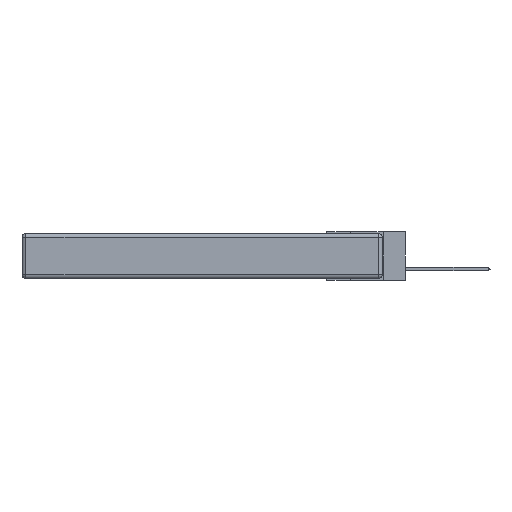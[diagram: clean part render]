
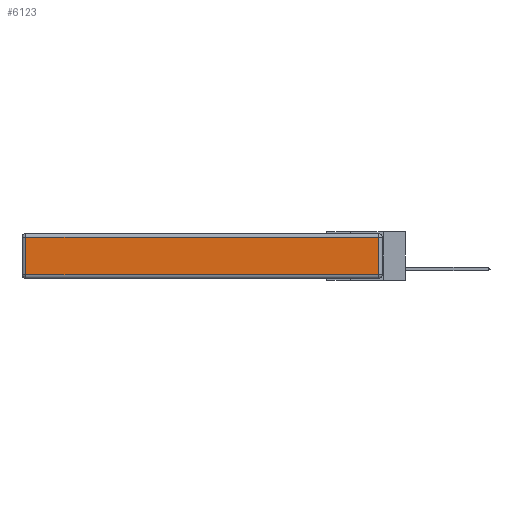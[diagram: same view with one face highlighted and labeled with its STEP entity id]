
A CAD part, left-side view. The second image highlights one B-rep face of the part: STEP entity #6123.
In plain terms, the highlighted planar face has unit normal (-1, 0, 0).
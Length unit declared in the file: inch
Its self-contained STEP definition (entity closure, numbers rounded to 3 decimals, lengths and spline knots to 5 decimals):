
#11 = AXIS2_PLACEMENT_3D ( 'NONE', #829, #14821, #4295 ) ;
#829 = CARTESIAN_POINT ( 'NONE',  ( 0., 0., -0.343 ) ) ;
#1125 = EDGE_LOOP ( 'NONE', ( #17814, #9909, #19989, #3002 ) ) ;
#2031 = VECTOR ( 'NONE', #16127, 39.37008 ) ;
#3002 = ORIENTED_EDGE ( 'NONE', *, *, #18448, .T. ) ;
#3499 = DIRECTION ( 'NONE',  ( 0., -1., 0. ) ) ;
#3679 = CARTESIAN_POINT ( 'NONE',  ( 0., 2.72, -0.313 ) ) ;
#4295 = DIRECTION ( 'NONE',  ( 0., 0., 1. ) ) ;
#5019 = EDGE_CURVE ( 'NONE', #17377, #13344, #14446, .T. ) ;
#5867 = PLANE ( 'NONE',  #11 ) ;
#6123 = ADVANCED_FACE ( 'NONE', ( #9942 ), #5867, .T. ) ;
#6393 = CARTESIAN_POINT ( 'NONE',  ( 0., 2.72, -0.03 ) ) ;
#8538 = VERTEX_POINT ( 'NONE', #3679 ) ;
#9721 = VECTOR ( 'NONE', #21737, 39.37008 ) ;
#9909 = ORIENTED_EDGE ( 'NONE', *, *, #11737, .T. ) ;
#9942 = FACE_OUTER_BOUND ( 'NONE', #1125, .T. ) ;
#10333 = CARTESIAN_POINT ( 'NONE',  ( 0., 2.72, -0.343 ) ) ;
#11701 = LINE ( 'NONE', #10333, #15592 ) ;
#11737 = EDGE_CURVE ( 'NONE', #16298, #17377, #13240, .T. ) ;
#13240 = LINE ( 'NONE', #17972, #2031 ) ;
#13344 = VERTEX_POINT ( 'NONE', #6393 ) ;
#14446 = LINE ( 'NONE', #14517, #9721 ) ;
#14517 = CARTESIAN_POINT ( 'NONE',  ( 0., 2.75, -0.03 ) ) ;
#14821 = DIRECTION ( 'NONE',  ( -1., 0., 0. ) ) ;
#15592 = VECTOR ( 'NONE', #15781, 39.37008 ) ;
#15781 = DIRECTION ( 'NONE',  ( 0., 0., -1. ) ) ;
#16127 = DIRECTION ( 'NONE',  ( 0., 0., 1. ) ) ;
#16257 = EDGE_CURVE ( 'NONE', #8538, #16298, #17781, .T. ) ;
#16298 = VERTEX_POINT ( 'NONE', #21259 ) ;
#17377 = VERTEX_POINT ( 'NONE', #18574 ) ;
#17781 = LINE ( 'NONE', #17916, #21116 ) ;
#17814 = ORIENTED_EDGE ( 'NONE', *, *, #16257, .T. ) ;
#17916 = CARTESIAN_POINT ( 'NONE',  ( 0., 0., -0.313 ) ) ;
#17972 = CARTESIAN_POINT ( 'NONE',  ( 0., 0.03, -0.343 ) ) ;
#18448 = EDGE_CURVE ( 'NONE', #13344, #8538, #11701, .T. ) ;
#18574 = CARTESIAN_POINT ( 'NONE',  ( 0., 0.03, -0.03 ) ) ;
#19989 = ORIENTED_EDGE ( 'NONE', *, *, #5019, .T. ) ;
#21116 = VECTOR ( 'NONE', #3499, 39.37008 ) ;
#21259 = CARTESIAN_POINT ( 'NONE',  ( 0., 0.03, -0.313 ) ) ;
#21737 = DIRECTION ( 'NONE',  ( 0., 1., 0. ) ) ;
